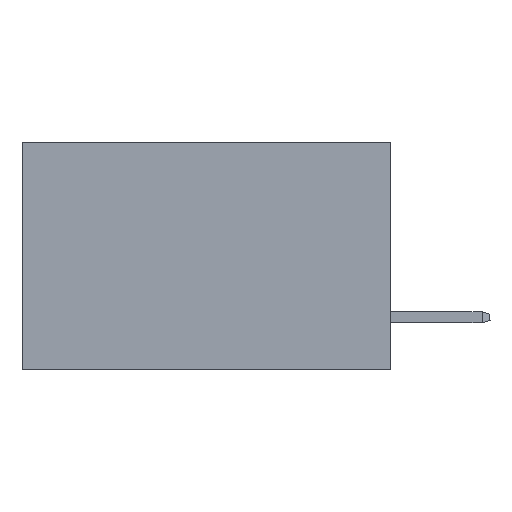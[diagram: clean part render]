
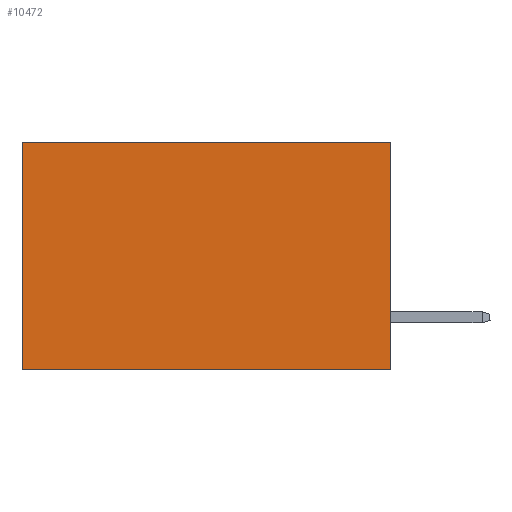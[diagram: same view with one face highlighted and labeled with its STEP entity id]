
A CAD part, left-side view. The second image highlights one B-rep face of the part: STEP entity #10472.
In plain terms, the highlighted planar face has unit normal (-1, 0, 0).
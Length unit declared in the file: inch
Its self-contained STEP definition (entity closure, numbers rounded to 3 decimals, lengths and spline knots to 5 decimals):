
#261 = DIRECTION ( 'NONE',  ( 0., 1., 0. ) ) ;
#303 = ORIENTED_EDGE ( 'NONE', *, *, #23930, .T. ) ;
#448 = EDGE_CURVE ( 'NONE', #19451, #9848, #8788, .T. ) ;
#2044 = EDGE_LOOP ( 'NONE', ( #8164, #9788, #5251, #303 ) ) ;
#2630 = CARTESIAN_POINT ( 'NONE',  ( 0.2875, 0.6, 0. ) ) ;
#2891 = AXIS2_PLACEMENT_3D ( 'NONE', #14736, #16717, #9386 ) ;
#4486 = VECTOR ( 'NONE', #5846, 39.37008 ) ;
#4793 = LINE ( 'NONE', #23279, #4486 ) ;
#5106 = VECTOR ( 'NONE', #13419, 39.37008 ) ;
#5251 = ORIENTED_EDGE ( 'NONE', *, *, #14286, .F. ) ;
#5846 = DIRECTION ( 'NONE',  ( 0., 1., 0. ) ) ;
#6493 = DIRECTION ( 'NONE',  ( 0., 0., -1. ) ) ;
#8164 = ORIENTED_EDGE ( 'NONE', *, *, #448, .T. ) ;
#8788 = LINE ( 'NONE', #25209, #5106 ) ;
#9128 = CARTESIAN_POINT ( 'NONE',  ( 0.2875, 0., 0. ) ) ;
#9386 = DIRECTION ( 'NONE',  ( 0., 0., -1. ) ) ;
#9788 = ORIENTED_EDGE ( 'NONE', *, *, #17183, .F. ) ;
#9848 = VERTEX_POINT ( 'NONE', #18391 ) ;
#10472 = ADVANCED_FACE ( 'NONE', ( #22560 ), #18743, .F. ) ;
#12538 = CARTESIAN_POINT ( 'NONE',  ( 0.2875, 0., 0. ) ) ;
#13163 = LINE ( 'NONE', #12538, #13739 ) ;
#13419 = DIRECTION ( 'NONE',  ( 0., 0., -1. ) ) ;
#13739 = VECTOR ( 'NONE', #6493, 39.37008 ) ;
#14286 = EDGE_CURVE ( 'NONE', #16986, #18952, #13163, .T. ) ;
#14736 = CARTESIAN_POINT ( 'NONE',  ( 0.2875, 0., 0. ) ) ;
#16669 = LINE ( 'NONE', #23502, #19682 ) ;
#16717 = DIRECTION ( 'NONE',  ( 1., 0., 0. ) ) ;
#16986 = VERTEX_POINT ( 'NONE', #9128 ) ;
#17183 = EDGE_CURVE ( 'NONE', #18952, #9848, #16669, .T. ) ;
#17431 = CARTESIAN_POINT ( 'NONE',  ( 0.2875, 0., -0.37 ) ) ;
#18391 = CARTESIAN_POINT ( 'NONE',  ( 0.2875, 0.6, -0.37 ) ) ;
#18743 = PLANE ( 'NONE',  #2891 ) ;
#18952 = VERTEX_POINT ( 'NONE', #17431 ) ;
#19451 = VERTEX_POINT ( 'NONE', #2630 ) ;
#19682 = VECTOR ( 'NONE', #261, 39.37008 ) ;
#22560 = FACE_OUTER_BOUND ( 'NONE', #2044, .T. ) ;
#23279 = CARTESIAN_POINT ( 'NONE',  ( 0.2875, 0., 0. ) ) ;
#23502 = CARTESIAN_POINT ( 'NONE',  ( 0.2875, 0., -0.37 ) ) ;
#23930 = EDGE_CURVE ( 'NONE', #16986, #19451, #4793, .T. ) ;
#25209 = CARTESIAN_POINT ( 'NONE',  ( 0.2875, 0.6, 0. ) ) ;
